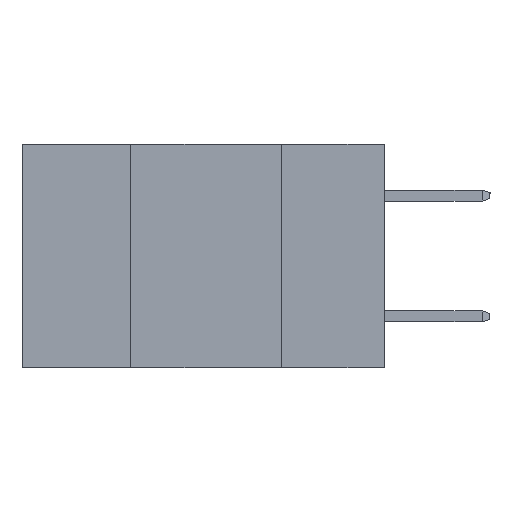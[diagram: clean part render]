
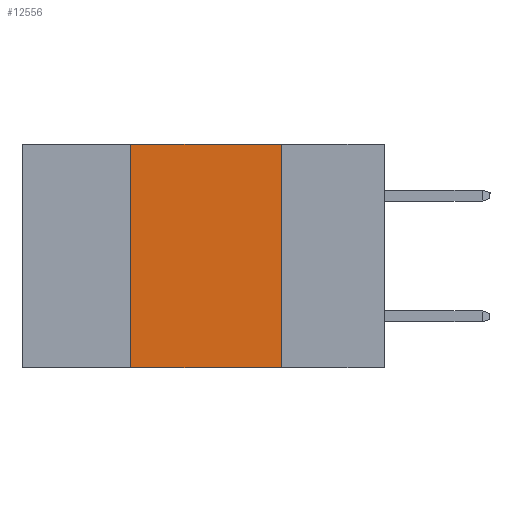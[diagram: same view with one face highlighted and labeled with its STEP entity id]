
A CAD part, left-side view. The second image highlights one B-rep face of the part: STEP entity #12556.
In plain terms, the highlighted planar face has unit normal (-1, 0, 0).
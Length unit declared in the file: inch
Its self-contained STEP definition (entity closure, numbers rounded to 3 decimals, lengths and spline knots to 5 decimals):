
#72 = CARTESIAN_POINT ( 'NONE',  ( 0., 0.42, 0. ) ) ;
#361 = LINE ( 'NONE', #10015, #4343 ) ;
#1126 = LINE ( 'NONE', #18859, #10168 ) ;
#1141 = ORIENTED_EDGE ( 'NONE', *, *, #11824, .F. ) ;
#1820 = CARTESIAN_POINT ( 'NONE',  ( 0., 0.6, 0. ) ) ;
#2324 = DIRECTION ( 'NONE',  ( 0., 0., -1. ) ) ;
#2611 = CARTESIAN_POINT ( 'NONE',  ( 0., 0.17, 0. ) ) ;
#3401 = FACE_OUTER_BOUND ( 'NONE', #18490, .T. ) ;
#4224 = VERTEX_POINT ( 'NONE', #16322 ) ;
#4343 = VECTOR ( 'NONE', #2324, 39.37008 ) ;
#4864 = CARTESIAN_POINT ( 'NONE',  ( 0., 0.6, -0.37 ) ) ;
#4980 = LINE ( 'NONE', #4864, #12963 ) ;
#5107 = ORIENTED_EDGE ( 'NONE', *, *, #15657, .F. ) ;
#5394 = VECTOR ( 'NONE', #6187, 39.37008 ) ;
#6187 = DIRECTION ( 'NONE',  ( 0., 0., 1. ) ) ;
#6233 = CARTESIAN_POINT ( 'NONE',  ( 0., 0.17, -0.37 ) ) ;
#6767 = DIRECTION ( 'NONE',  ( 0., -1., 0. ) ) ;
#8714 = VERTEX_POINT ( 'NONE', #6233 ) ;
#10015 = CARTESIAN_POINT ( 'NONE',  ( 0., 0.17, -0.37 ) ) ;
#10168 = VECTOR ( 'NONE', #6767, 39.37008 ) ;
#11339 = PLANE ( 'NONE',  #21783 ) ;
#11824 = EDGE_CURVE ( 'NONE', #4224, #21435, #12545, .T. ) ;
#12033 = CARTESIAN_POINT ( 'NONE',  ( 0., 0.42, -0.37 ) ) ;
#12545 = LINE ( 'NONE', #12033, #5394 ) ;
#12556 = ADVANCED_FACE ( 'NONE', ( #3401 ), #11339, .F. ) ;
#12627 = ORIENTED_EDGE ( 'NONE', *, *, #15037, .F. ) ;
#12963 = VECTOR ( 'NONE', #20467, 39.37008 ) ;
#15037 = EDGE_CURVE ( 'NONE', #18493, #8714, #361, .T. ) ;
#15657 = EDGE_CURVE ( 'NONE', #21435, #18493, #1126, .T. ) ;
#15899 = ORIENTED_EDGE ( 'NONE', *, *, #25198, .T. ) ;
#16322 = CARTESIAN_POINT ( 'NONE',  ( 0., 0.42, -0.37 ) ) ;
#18490 = EDGE_LOOP ( 'NONE', ( #12627, #5107, #1141, #15899 ) ) ;
#18493 = VERTEX_POINT ( 'NONE', #2611 ) ;
#18859 = CARTESIAN_POINT ( 'NONE',  ( 0., 0.6, 0. ) ) ;
#19293 = DIRECTION ( 'NONE',  ( 0., 0., -1. ) ) ;
#20467 = DIRECTION ( 'NONE',  ( 0., -1., 0. ) ) ;
#21435 = VERTEX_POINT ( 'NONE', #72 ) ;
#21783 = AXIS2_PLACEMENT_3D ( 'NONE', #1820, #23576, #19293 ) ;
#23576 = DIRECTION ( 'NONE',  ( 1., 0., 0. ) ) ;
#25198 = EDGE_CURVE ( 'NONE', #4224, #8714, #4980, .T. ) ;
